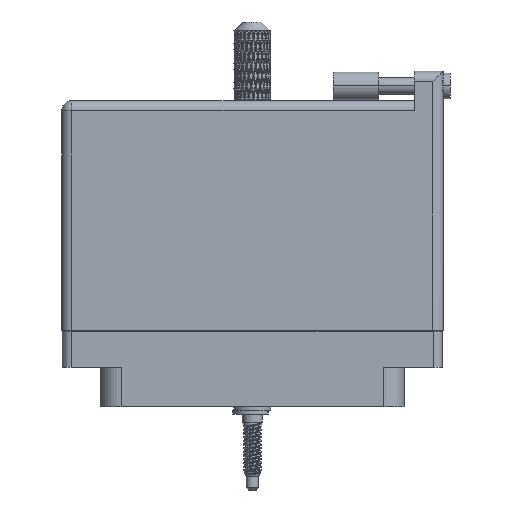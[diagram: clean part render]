
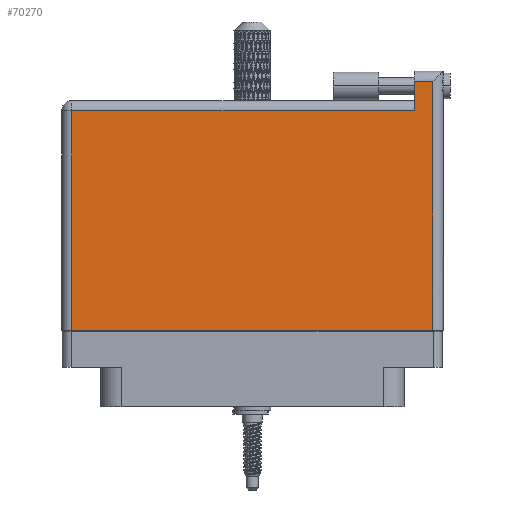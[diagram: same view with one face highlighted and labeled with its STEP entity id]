
A CAD part, front view. The second image highlights one B-rep face of the part: STEP entity #70270.
In plain terms, the highlighted face is planar.
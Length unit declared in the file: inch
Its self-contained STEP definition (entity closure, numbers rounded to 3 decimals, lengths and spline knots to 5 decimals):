
#6216 = ORIENTED_EDGE ( 'NONE', *, *, #96653, .T. ) ;
#10251 = LINE ( 'NONE', #28851, #42851 ) ;
#15258 = EDGE_CURVE ( 'NONE', #55854, #103870, #35814, .T. ) ;
#18849 = CARTESIAN_POINT ( 'NONE',  ( -1.23, -0.1, 0.4495 ) ) ;
#19546 = ORIENTED_EDGE ( 'NONE', *, *, #108281, .T. ) ;
#25195 = EDGE_CURVE ( 'NONE', #83493, #55854, #10251, .T. ) ;
#25798 = CARTESIAN_POINT ( 'NONE',  ( 1.103, 1.596, 0.4495 ) ) ;
#27296 = ORIENTED_EDGE ( 'NONE', *, *, #25195, .T. ) ;
#28184 = CARTESIAN_POINT ( 'NONE',  ( 1.103, 1.666, 0.4495 ) ) ;
#28851 = CARTESIAN_POINT ( 'NONE',  ( 1.23, 1.666, 0.4495 ) ) ;
#32357 = VECTOR ( 'NONE', #79340, 39.37008 ) ;
#32552 = CARTESIAN_POINT ( 'NONE',  ( -1.3, -0.1, 0.4495 ) ) ;
#33707 = ORIENTED_EDGE ( 'NONE', *, *, #15258, .T. ) ;
#34704 = CARTESIAN_POINT ( 'NONE',  ( -1.3, 1.466, 0.4495 ) ) ;
#35814 = LINE ( 'NONE', #113361, #68367 ) ;
#36518 = DIRECTION ( 'NONE',  ( 0., -1., 0. ) ) ;
#37967 = VECTOR ( 'NONE', #36518, 39.37008 ) ;
#42851 = VECTOR ( 'NONE', #64863, 39.37008 ) ;
#43768 = DIRECTION ( 'NONE',  ( 0., 0., -1. ) ) ;
#44008 = LINE ( 'NONE', #32552, #53911 ) ;
#44543 = DIRECTION ( 'NONE',  ( 0., -1., 0. ) ) ;
#48704 = FACE_OUTER_BOUND ( 'NONE', #114999, .T. ) ;
#51762 = ORIENTED_EDGE ( 'NONE', *, *, #92011, .T. ) ;
#52496 = DIRECTION ( 'NONE',  ( -1., 0., 0. ) ) ;
#53235 = AXIS2_PLACEMENT_3D ( 'NONE', #34704, #43768, #52496 ) ;
#53911 = VECTOR ( 'NONE', #98278, 39.37008 ) ;
#55854 = VERTEX_POINT ( 'NONE', #89372 ) ;
#61064 = CARTESIAN_POINT ( 'NONE',  ( -1.3, 1.396, 0.4495 ) ) ;
#61881 = LINE ( 'NONE', #18849, #101633 ) ;
#64863 = DIRECTION ( 'NONE',  ( 0., 1., 0. ) ) ;
#68367 = VECTOR ( 'NONE', #86452, 39.37008 ) ;
#70270 = ADVANCED_FACE ( 'NONE', ( #48704 ), #70314, .F. ) ;
#70314 = PLANE ( 'NONE',  #53235 ) ;
#74013 = VERTEX_POINT ( 'NONE', #87412 ) ;
#76174 = VERTEX_POINT ( 'NONE', #79253 ) ;
#79253 = CARTESIAN_POINT ( 'NONE',  ( -1.23, 1.396, 0.4495 ) ) ;
#79340 = DIRECTION ( 'NONE',  ( -1., 0., 0. ) ) ;
#83493 = VERTEX_POINT ( 'NONE', #107466 ) ;
#84782 = LINE ( 'NONE', #61064, #32357 ) ;
#86452 = DIRECTION ( 'NONE',  ( -1., 0., 0. ) ) ;
#87412 = CARTESIAN_POINT ( 'NONE',  ( 1.103, 1.396, 0.4495 ) ) ;
#89372 = CARTESIAN_POINT ( 'NONE',  ( 1.23, 1.596, 0.4495 ) ) ;
#92011 = EDGE_CURVE ( 'NONE', #95183, #83493, #44008, .T. ) ;
#95183 = VERTEX_POINT ( 'NONE', #110429 ) ;
#96653 = EDGE_CURVE ( 'NONE', #76174, #95183, #61881, .T. ) ;
#98278 = DIRECTION ( 'NONE',  ( 1., 0., 0. ) ) ;
#98959 = LINE ( 'NONE', #28184, #37967 ) ;
#101633 = VECTOR ( 'NONE', #44543, 39.37008 ) ;
#103870 = VERTEX_POINT ( 'NONE', #25798 ) ;
#104527 = ORIENTED_EDGE ( 'NONE', *, *, #108169, .T. ) ;
#107466 = CARTESIAN_POINT ( 'NONE',  ( 1.23, -0.1, 0.4495 ) ) ;
#108169 = EDGE_CURVE ( 'NONE', #74013, #76174, #84782, .T. ) ;
#108281 = EDGE_CURVE ( 'NONE', #103870, #74013, #98959, .T. ) ;
#110429 = CARTESIAN_POINT ( 'NONE',  ( -1.23, -0.1, 0.4495 ) ) ;
#113361 = CARTESIAN_POINT ( 'NONE',  ( -1.3, 1.596, 0.4495 ) ) ;
#114999 = EDGE_LOOP ( 'NONE', ( #51762, #27296, #33707, #19546, #104527, #6216 ) ) ;
